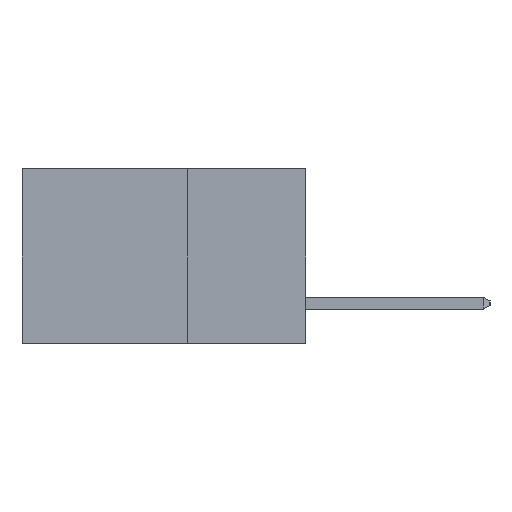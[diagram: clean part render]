
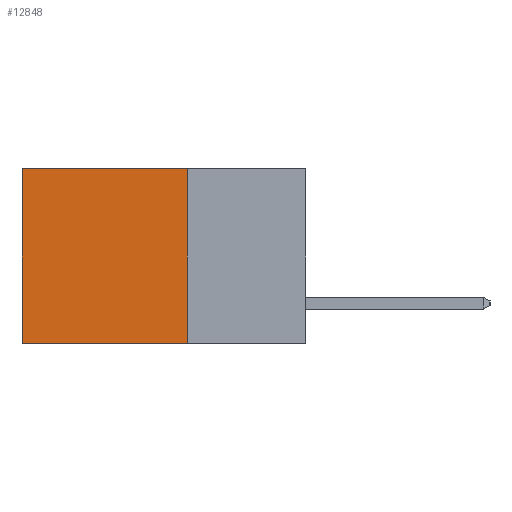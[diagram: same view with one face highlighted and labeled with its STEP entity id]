
A CAD part, left-side view. The second image highlights one B-rep face of the part: STEP entity #12848.
In plain terms, the highlighted planar face has unit normal (-1, 0, 0).
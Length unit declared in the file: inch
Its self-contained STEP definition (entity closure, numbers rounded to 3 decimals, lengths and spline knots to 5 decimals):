
#364 = LINE ( 'NONE', #6975, #22415 ) ;
#2431 = VECTOR ( 'NONE', #17640, 39.37008 ) ;
#2581 = CARTESIAN_POINT ( 'NONE',  ( 0.2615, 0.25, -0.37 ) ) ;
#3364 = DIRECTION ( 'NONE',  ( 0., 0., -1. ) ) ;
#3418 = DIRECTION ( 'NONE',  ( 1., 0., 0. ) ) ;
#3475 = CARTESIAN_POINT ( 'NONE',  ( 0.2615, 0.25, -0.37 ) ) ;
#3572 = PLANE ( 'NONE',  #3872 ) ;
#3872 = AXIS2_PLACEMENT_3D ( 'NONE', #3475, #3418, #3364 ) ;
#6747 = DIRECTION ( 'NONE',  ( 0., 1., 0. ) ) ;
#6975 = CARTESIAN_POINT ( 'NONE',  ( 0.2615, 0.25, 0. ) ) ;
#7341 = CARTESIAN_POINT ( 'NONE',  ( 0.2615, 0.6, 0. ) ) ;
#7551 = EDGE_CURVE ( 'NONE', #19413, #11578, #364, .T. ) ;
#7802 = LINE ( 'NONE', #15939, #2431 ) ;
#9120 = LINE ( 'NONE', #2581, #13823 ) ;
#11578 = VERTEX_POINT ( 'NONE', #7341 ) ;
#11900 = VECTOR ( 'NONE', #13939, 39.37008 ) ;
#12209 = CARTESIAN_POINT ( 'NONE',  ( 0.2615, 0.25, -0.37 ) ) ;
#12253 = CARTESIAN_POINT ( 'NONE',  ( 0.2615, 0.6, -0.37 ) ) ;
#12807 = ORIENTED_EDGE ( 'NONE', *, *, #16127, .F. ) ;
#12848 = ADVANCED_FACE ( 'NONE', ( #15774 ), #3572, .F. ) ;
#13259 = CARTESIAN_POINT ( 'NONE',  ( 0.2615, 0.25, -0.37 ) ) ;
#13823 = VECTOR ( 'NONE', #20034, 39.37008 ) ;
#13939 = DIRECTION ( 'NONE',  ( 0., 1., 0. ) ) ;
#14700 = ORIENTED_EDGE ( 'NONE', *, *, #19894, .F. ) ;
#14784 = ORIENTED_EDGE ( 'NONE', *, *, #7551, .T. ) ;
#15774 = FACE_OUTER_BOUND ( 'NONE', #20360, .T. ) ;
#15939 = CARTESIAN_POINT ( 'NONE',  ( 0.2615, 0.6, -0.37 ) ) ;
#16127 = EDGE_CURVE ( 'NONE', #18364, #18626, #20887, .T. ) ;
#17640 = DIRECTION ( 'NONE',  ( 0., 0., -1. ) ) ;
#18094 = EDGE_CURVE ( 'NONE', #11578, #18626, #7802, .T. ) ;
#18364 = VERTEX_POINT ( 'NONE', #13259 ) ;
#18626 = VERTEX_POINT ( 'NONE', #12253 ) ;
#19413 = VERTEX_POINT ( 'NONE', #21762 ) ;
#19439 = ORIENTED_EDGE ( 'NONE', *, *, #18094, .T. ) ;
#19894 = EDGE_CURVE ( 'NONE', #19413, #18364, #9120, .T. ) ;
#20034 = DIRECTION ( 'NONE',  ( 0., 0., -1. ) ) ;
#20360 = EDGE_LOOP ( 'NONE', ( #19439, #12807, #14700, #14784 ) ) ;
#20887 = LINE ( 'NONE', #12209, #11900 ) ;
#21762 = CARTESIAN_POINT ( 'NONE',  ( 0.2615, 0.25, 0. ) ) ;
#22415 = VECTOR ( 'NONE', #6747, 39.37008 ) ;
